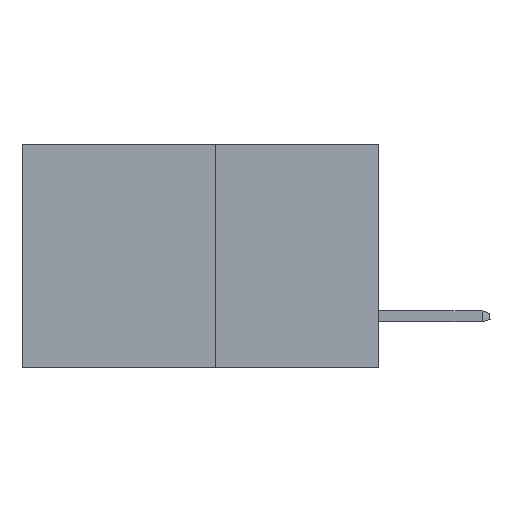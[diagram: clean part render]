
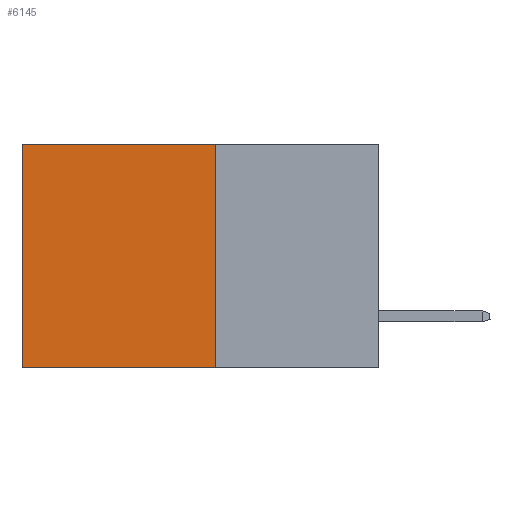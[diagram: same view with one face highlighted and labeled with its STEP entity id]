
A CAD part, left-side view. The second image highlights one B-rep face of the part: STEP entity #6145.
In plain terms, the highlighted planar face has unit normal (-1, 0, 0).
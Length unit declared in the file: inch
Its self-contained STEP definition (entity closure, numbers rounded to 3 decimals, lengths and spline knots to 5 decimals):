
#654 = EDGE_CURVE ( 'NONE', #5388, #8398, #2907, .T. ) ;
#1497 = EDGE_CURVE ( 'NONE', #5388, #6505, #11733, .T. ) ;
#1836 = DIRECTION ( 'NONE',  ( 0., 0., -1. ) ) ;
#2047 = CARTESIAN_POINT ( 'NONE',  ( 0.277, 0.59, 0. ) ) ;
#2371 = CARTESIAN_POINT ( 'NONE',  ( 0.277, 0.27, -0.37 ) ) ;
#2534 = CARTESIAN_POINT ( 'NONE',  ( 0.277, 0.27, -0.37 ) ) ;
#2756 = CARTESIAN_POINT ( 'NONE',  ( 0.277, 0.59, -0.37 ) ) ;
#2907 = LINE ( 'NONE', #11392, #5278 ) ;
#2914 = ORIENTED_EDGE ( 'NONE', *, *, #10791, .F. ) ;
#3053 = AXIS2_PLACEMENT_3D ( 'NONE', #2534, #5578, #12449 ) ;
#3545 = VECTOR ( 'NONE', #5863, 39.37008 ) ;
#3565 = PLANE ( 'NONE',  #3053 ) ;
#4638 = EDGE_LOOP ( 'NONE', ( #8711, #2914, #5934, #9461 ) ) ;
#5278 = VECTOR ( 'NONE', #1836, 39.37008 ) ;
#5388 = VERTEX_POINT ( 'NONE', #12134 ) ;
#5578 = DIRECTION ( 'NONE',  ( 1., 0., 0. ) ) ;
#5859 = EDGE_CURVE ( 'NONE', #6505, #10493, #12686, .T. ) ;
#5863 = DIRECTION ( 'NONE',  ( 0., 1., 0. ) ) ;
#5934 = ORIENTED_EDGE ( 'NONE', *, *, #654, .F. ) ;
#6145 = ADVANCED_FACE ( 'NONE', ( #9926 ), #3565, .F. ) ;
#6505 = VERTEX_POINT ( 'NONE', #2047 ) ;
#6609 = VECTOR ( 'NONE', #12163, 39.37008 ) ;
#7262 = CARTESIAN_POINT ( 'NONE',  ( 0.277, 0.27, -0.37 ) ) ;
#8014 = CARTESIAN_POINT ( 'NONE',  ( 0.277, 0.27, 0. ) ) ;
#8101 = CARTESIAN_POINT ( 'NONE',  ( 0.277, 0.59, -0.37 ) ) ;
#8398 = VERTEX_POINT ( 'NONE', #2371 ) ;
#8711 = ORIENTED_EDGE ( 'NONE', *, *, #5859, .T. ) ;
#9461 = ORIENTED_EDGE ( 'NONE', *, *, #1497, .T. ) ;
#9926 = FACE_OUTER_BOUND ( 'NONE', #4638, .T. ) ;
#10090 = VECTOR ( 'NONE', #11029, 39.37008 ) ;
#10493 = VERTEX_POINT ( 'NONE', #2756 ) ;
#10791 = EDGE_CURVE ( 'NONE', #8398, #10493, #11518, .T. ) ;
#11029 = DIRECTION ( 'NONE',  ( 0., 0., -1. ) ) ;
#11392 = CARTESIAN_POINT ( 'NONE',  ( 0.277, 0.27, -0.37 ) ) ;
#11518 = LINE ( 'NONE', #7262, #6609 ) ;
#11733 = LINE ( 'NONE', #8014, #3545 ) ;
#12134 = CARTESIAN_POINT ( 'NONE',  ( 0.277, 0.27, 0. ) ) ;
#12163 = DIRECTION ( 'NONE',  ( 0., 1., 0. ) ) ;
#12449 = DIRECTION ( 'NONE',  ( 0., 0., -1. ) ) ;
#12686 = LINE ( 'NONE', #8101, #10090 ) ;
